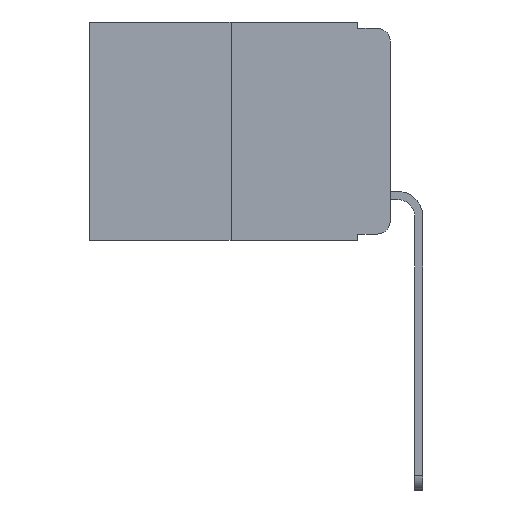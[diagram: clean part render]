
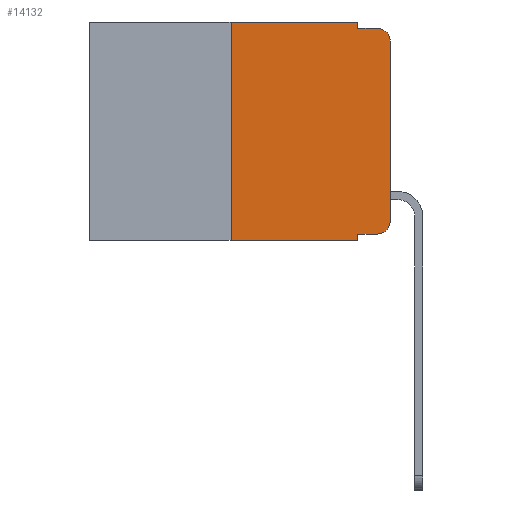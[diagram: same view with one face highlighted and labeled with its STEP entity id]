
A CAD part, left-side view. The second image highlights one B-rep face of the part: STEP entity #14132.
In plain terms, the highlighted planar face has unit normal (-1, 0, 0).
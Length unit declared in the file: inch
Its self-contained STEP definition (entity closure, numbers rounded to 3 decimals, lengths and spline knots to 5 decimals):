
#72 = AXIS2_PLACEMENT_3D ( 'NONE', #21040, #4710, #16420 ) ;
#307 = LINE ( 'NONE', #17530, #9396 ) ;
#361 = CARTESIAN_POINT ( 'NONE',  ( 0., 0.051, 0. ) ) ;
#629 = CARTESIAN_POINT ( 'NONE',  ( 0., 0.02, -0.01 ) ) ;
#892 = LINE ( 'NONE', #12346, #14756 ) ;
#1168 = DIRECTION ( 'NONE',  ( 0., -1., 0. ) ) ;
#1454 = ORIENTED_EDGE ( 'NONE', *, *, #8456, .F. ) ;
#1525 = VECTOR ( 'NONE', #1777, 39.37008 ) ;
#1778 = CARTESIAN_POINT ( 'NONE',  ( 0., 0., -0.03 ) ) ;
#1777 = DIRECTION ( 'NONE',  ( 0., 0., -1. ) ) ;
#2222 = CARTESIAN_POINT ( 'NONE',  ( 0., 0.02, -0.333 ) ) ;
#2300 = DIRECTION ( 'NONE',  ( 0., 0., -1. ) ) ;
#2465 = VERTEX_POINT ( 'NONE', #1778 ) ;
#3121 = CARTESIAN_POINT ( 'NONE',  ( 0., 0.473, -0.343 ) ) ;
#3550 = DIRECTION ( 'NONE',  ( 0., 0., 1. ) ) ;
#3643 = CARTESIAN_POINT ( 'NONE',  ( 0., 0.25, 0. ) ) ;
#4450 = ORIENTED_EDGE ( 'NONE', *, *, #10340, .T. ) ;
#4585 = VERTEX_POINT ( 'NONE', #5903 ) ;
#4710 = DIRECTION ( 'NONE',  ( 1., 0., 0. ) ) ;
#5023 = ORIENTED_EDGE ( 'NONE', *, *, #10375, .T. ) ;
#5903 = CARTESIAN_POINT ( 'NONE',  ( 0., 0.25, 0. ) ) ;
#5941 = AXIS2_PLACEMENT_3D ( 'NONE', #7451, #18870, #9137 ) ;
#6059 = VERTEX_POINT ( 'NONE', #14372 ) ;
#6376 = AXIS2_PLACEMENT_3D ( 'NONE', #19036, #9326, #20564 ) ;
#6504 = CIRCLE ( 'NONE', #6376, 0.02 ) ;
#6897 = CARTESIAN_POINT ( 'NONE',  ( 0., 0., -0.313 ) ) ;
#7451 = CARTESIAN_POINT ( 'NONE',  ( 0., 0.02, -0.313 ) ) ;
#7658 = CARTESIAN_POINT ( 'NONE',  ( 0., 0.25, -0.343 ) ) ;
#7970 = CARTESIAN_POINT ( 'NONE',  ( 0., 0.051, -0.01 ) ) ;
#8016 = ORIENTED_EDGE ( 'NONE', *, *, #9893, .T. ) ;
#8227 = DIRECTION ( 'NONE',  ( 0., -1., 0. ) ) ;
#8456 = EDGE_CURVE ( 'NONE', #4585, #15729, #11451, .T. ) ;
#8764 = LINE ( 'NONE', #3121, #16992 ) ;
#8863 = LINE ( 'NONE', #361, #12756 ) ;
#9137 = DIRECTION ( 'NONE',  ( 0., 0., -1. ) ) ;
#9251 = EDGE_CURVE ( 'NONE', #9506, #13594, #8764, .T. ) ;
#9326 = DIRECTION ( 'NONE',  ( -1., 0., 0. ) ) ;
#9396 = VECTOR ( 'NONE', #12649, 39.37008 ) ;
#9506 = VERTEX_POINT ( 'NONE', #7658 ) ;
#9893 = EDGE_CURVE ( 'NONE', #11695, #2465, #9962, .T. ) ;
#9895 = EDGE_CURVE ( 'NONE', #2465, #15264, #6504, .T. ) ;
#9938 = EDGE_CURVE ( 'NONE', #20631, #15264, #307, .T. ) ;
#9962 = LINE ( 'NONE', #14183, #18032 ) ;
#9969 = EDGE_CURVE ( 'NONE', #15729, #20631, #8863, .T. ) ;
#10310 = EDGE_CURVE ( 'NONE', #9506, #4585, #15801, .T. ) ;
#10314 = EDGE_CURVE ( 'NONE', #6059, #13594, #19487, .T. ) ;
#10340 = EDGE_CURVE ( 'NONE', #6059, #13270, #892, .T. ) ;
#10375 = EDGE_CURVE ( 'NONE', #13270, #11695, #18305, .T. ) ;
#10639 = CARTESIAN_POINT ( 'NONE',  ( 0., 0.051, 0. ) ) ;
#11421 = ORIENTED_EDGE ( 'NONE', *, *, #10310, .F. ) ;
#11451 = LINE ( 'NONE', #16447, #15251 ) ;
#11695 = VERTEX_POINT ( 'NONE', #6897 ) ;
#12185 = CARTESIAN_POINT ( 'NONE',  ( 0., 0.051, 0. ) ) ;
#12346 = CARTESIAN_POINT ( 'NONE',  ( 0., 0.051, -0.333 ) ) ;
#12438 = ORIENTED_EDGE ( 'NONE', *, *, #9251, .T. ) ;
#12587 = DIRECTION ( 'NONE',  ( 0., 0., 1. ) ) ;
#12649 = DIRECTION ( 'NONE',  ( 0., -1., 0. ) ) ;
#12756 = VECTOR ( 'NONE', #2300, 39.37008 ) ;
#13180 = CARTESIAN_POINT ( 'NONE',  ( 0., 0.051, -0.343 ) ) ;
#13270 = VERTEX_POINT ( 'NONE', #2222 ) ;
#13594 = VERTEX_POINT ( 'NONE', #13180 ) ;
#14132 = ADVANCED_FACE ( 'NONE', ( #19234 ), #19490, .F. ) ;
#14183 = CARTESIAN_POINT ( 'NONE',  ( 0., 0., 0. ) ) ;
#14372 = CARTESIAN_POINT ( 'NONE',  ( 0., 0.051, -0.333 ) ) ;
#14474 = ORIENTED_EDGE ( 'NONE', *, *, #9969, .F. ) ;
#14756 = VECTOR ( 'NONE', #21802, 39.37008 ) ;
#15251 = VECTOR ( 'NONE', #8227, 39.37008 ) ;
#15264 = VERTEX_POINT ( 'NONE', #629 ) ;
#15281 = VECTOR ( 'NONE', #3550, 39.37008 ) ;
#15729 = VERTEX_POINT ( 'NONE', #12185 ) ;
#15801 = LINE ( 'NONE', #3643, #15281 ) ;
#15959 = EDGE_LOOP ( 'NONE', ( #8016, #21857, #18240, #14474, #1454, #11421, #12438, #16768, #4450, #5023 ) ) ;
#16420 = DIRECTION ( 'NONE',  ( 0., 0., -1. ) ) ;
#16447 = CARTESIAN_POINT ( 'NONE',  ( 0., 0.473, 0. ) ) ;
#16768 = ORIENTED_EDGE ( 'NONE', *, *, #10314, .F. ) ;
#16992 = VECTOR ( 'NONE', #1168, 39.37008 ) ;
#17530 = CARTESIAN_POINT ( 'NONE',  ( 0., 0.051, -0.01 ) ) ;
#18032 = VECTOR ( 'NONE', #12587, 39.37008 ) ;
#18240 = ORIENTED_EDGE ( 'NONE', *, *, #9938, .F. ) ;
#18305 = CIRCLE ( 'NONE', #5941, 0.02 ) ;
#18870 = DIRECTION ( 'NONE',  ( -1., 0., 0. ) ) ;
#19036 = CARTESIAN_POINT ( 'NONE',  ( 0., 0.02, -0.03 ) ) ;
#19234 = FACE_OUTER_BOUND ( 'NONE', #15959, .T. ) ;
#19487 = LINE ( 'NONE', #10639, #1525 ) ;
#19490 = PLANE ( 'NONE',  #72 ) ;
#20564 = DIRECTION ( 'NONE',  ( 0., 0., -1. ) ) ;
#20631 = VERTEX_POINT ( 'NONE', #7970 ) ;
#21040 = CARTESIAN_POINT ( 'NONE',  ( 0., 0.473, 0. ) ) ;
#21802 = DIRECTION ( 'NONE',  ( 0., -1., 0. ) ) ;
#21857 = ORIENTED_EDGE ( 'NONE', *, *, #9895, .T. ) ;
